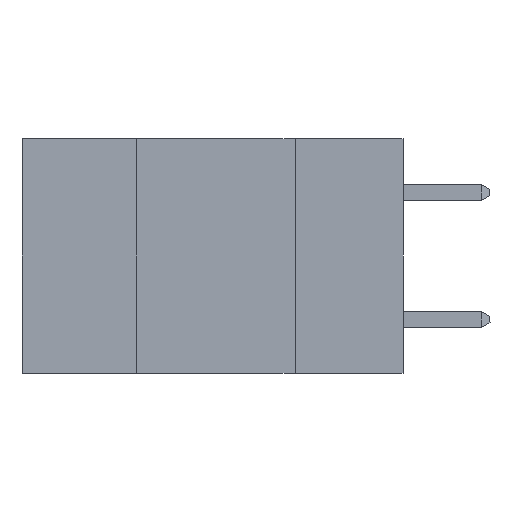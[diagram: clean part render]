
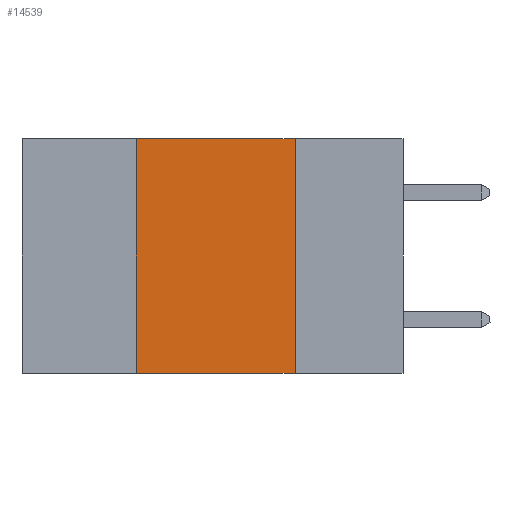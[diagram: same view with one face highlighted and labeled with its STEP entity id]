
A CAD part, left-side view. The second image highlights one B-rep face of the part: STEP entity #14539.
In plain terms, the highlighted planar face has unit normal (-1, 0, 0).
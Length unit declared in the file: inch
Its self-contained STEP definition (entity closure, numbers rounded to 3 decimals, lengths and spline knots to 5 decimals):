
#133 = DIRECTION ( 'NONE',  ( 0., 0., -1. ) ) ;
#737 = DIRECTION ( 'NONE',  ( 0., 0., -1. ) ) ;
#1345 = LINE ( 'NONE', #2064, #14493 ) ;
#1958 = VERTEX_POINT ( 'NONE', #14017 ) ;
#2064 = CARTESIAN_POINT ( 'NONE',  ( 0., 0.6, -0.37 ) ) ;
#2982 = EDGE_CURVE ( 'NONE', #1958, #13873, #1345, .T. ) ;
#3088 = EDGE_CURVE ( 'NONE', #1958, #3589, #15080, .T. ) ;
#3589 = VERTEX_POINT ( 'NONE', #4182 ) ;
#3750 = ORIENTED_EDGE ( 'NONE', *, *, #13894, .F. ) ;
#3792 = ORIENTED_EDGE ( 'NONE', *, *, #2982, .T. ) ;
#3993 = FACE_OUTER_BOUND ( 'NONE', #11360, .T. ) ;
#4182 = CARTESIAN_POINT ( 'NONE',  ( 0., 0.42, 0. ) ) ;
#4469 = CARTESIAN_POINT ( 'NONE',  ( 0., 0.17, 0. ) ) ;
#6155 = DIRECTION ( 'NONE',  ( 0., 0., 1. ) ) ;
#6183 = VECTOR ( 'NONE', #7231, 39.37008 ) ;
#7231 = DIRECTION ( 'NONE',  ( 0., -1., 0. ) ) ;
#7365 = CARTESIAN_POINT ( 'NONE',  ( 0., 0.17, 0. ) ) ;
#7480 = CARTESIAN_POINT ( 'NONE',  ( 0., 0.6, 0. ) ) ;
#8326 = LINE ( 'NONE', #13492, #6183 ) ;
#8950 = EDGE_CURVE ( 'NONE', #13445, #13873, #12039, .T. ) ;
#9335 = PLANE ( 'NONE',  #14351 ) ;
#11053 = DIRECTION ( 'NONE',  ( 0., -1., 0. ) ) ;
#11360 = EDGE_LOOP ( 'NONE', ( #13559, #3750, #12270, #3792 ) ) ;
#12039 = LINE ( 'NONE', #4469, #14926 ) ;
#12270 = ORIENTED_EDGE ( 'NONE', *, *, #3088, .F. ) ;
#13445 = VERTEX_POINT ( 'NONE', #7365 ) ;
#13492 = CARTESIAN_POINT ( 'NONE',  ( 0., 0.6, 0. ) ) ;
#13519 = VECTOR ( 'NONE', #6155, 39.37008 ) ;
#13559 = ORIENTED_EDGE ( 'NONE', *, *, #8950, .F. ) ;
#13873 = VERTEX_POINT ( 'NONE', #14347 ) ;
#13894 = EDGE_CURVE ( 'NONE', #3589, #13445, #8326, .T. ) ;
#14017 = CARTESIAN_POINT ( 'NONE',  ( 0., 0.42, -0.37 ) ) ;
#14347 = CARTESIAN_POINT ( 'NONE',  ( 0., 0.17, -0.37 ) ) ;
#14351 = AXIS2_PLACEMENT_3D ( 'NONE', #7480, #15092, #133 ) ;
#14493 = VECTOR ( 'NONE', #11053, 39.37008 ) ;
#14539 = ADVANCED_FACE ( 'NONE', ( #3993 ), #9335, .F. ) ;
#14926 = VECTOR ( 'NONE', #737, 39.37008 ) ;
#15080 = LINE ( 'NONE', #16039, #13519 ) ;
#15092 = DIRECTION ( 'NONE',  ( 1., 0., 0. ) ) ;
#16039 = CARTESIAN_POINT ( 'NONE',  ( 0., 0.42, 0. ) ) ;
